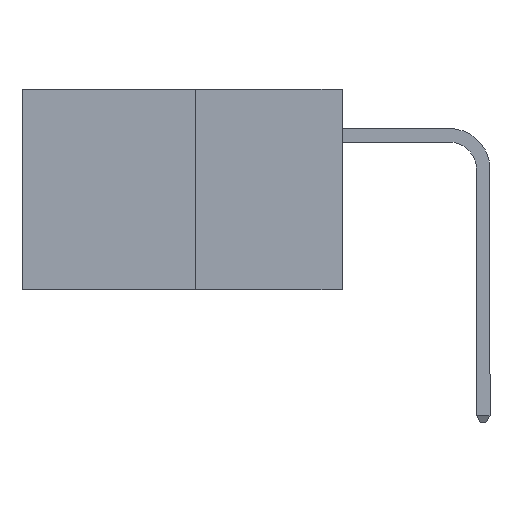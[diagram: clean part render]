
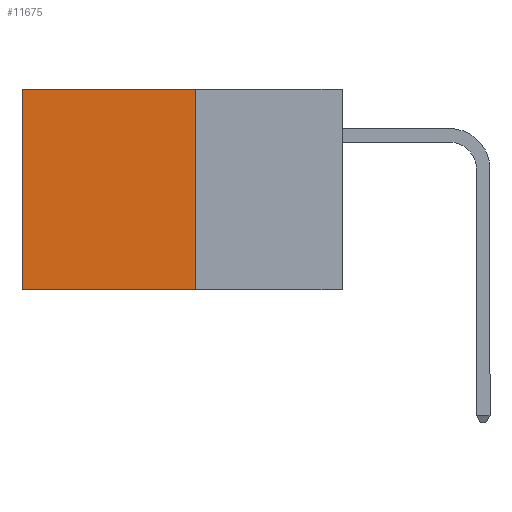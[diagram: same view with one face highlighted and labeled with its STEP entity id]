
A CAD part, left-side view. The second image highlights one B-rep face of the part: STEP entity #11675.
In plain terms, the highlighted planar face has unit normal (-1, 0, 0).
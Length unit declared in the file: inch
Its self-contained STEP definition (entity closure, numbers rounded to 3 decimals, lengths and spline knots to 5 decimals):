
#124 = LINE ( 'NONE', #11530, #7483 ) ;
#128 = CARTESIAN_POINT ( 'NONE',  ( 0.277, 0.59, -0.37 ) ) ;
#208 = VERTEX_POINT ( 'NONE', #7636 ) ;
#1012 = CARTESIAN_POINT ( 'NONE',  ( 0.277, 0.59, 0. ) ) ;
#1366 = ORIENTED_EDGE ( 'NONE', *, *, #8834, .T. ) ;
#1593 = CARTESIAN_POINT ( 'NONE',  ( 0.277, 0.27, -0.37 ) ) ;
#1611 = DIRECTION ( 'NONE',  ( 0., 1., 0. ) ) ;
#2926 = DIRECTION ( 'NONE',  ( 0., 0., -1. ) ) ;
#3081 = VERTEX_POINT ( 'NONE', #1012 ) ;
#3331 = ORIENTED_EDGE ( 'NONE', *, *, #4728, .F. ) ;
#4112 = DIRECTION ( 'NONE',  ( 0., 0., -1. ) ) ;
#4430 = FACE_OUTER_BOUND ( 'NONE', #7140, .T. ) ;
#4728 = EDGE_CURVE ( 'NONE', #208, #9255, #12239, .T. ) ;
#5183 = EDGE_CURVE ( 'NONE', #6475, #208, #7629, .T. ) ;
#5600 = ORIENTED_EDGE ( 'NONE', *, *, #7944, .T. ) ;
#5787 = CARTESIAN_POINT ( 'NONE',  ( 0.277, 0.27, 0. ) ) ;
#6002 = AXIS2_PLACEMENT_3D ( 'NONE', #6958, #9772, #4112 ) ;
#6021 = PLANE ( 'NONE',  #6002 ) ;
#6188 = ORIENTED_EDGE ( 'NONE', *, *, #5183, .F. ) ;
#6475 = VERTEX_POINT ( 'NONE', #5787 ) ;
#6736 = CARTESIAN_POINT ( 'NONE',  ( 0.277, 0.27, -0.37 ) ) ;
#6958 = CARTESIAN_POINT ( 'NONE',  ( 0.277, 0.27, -0.37 ) ) ;
#7140 = EDGE_LOOP ( 'NONE', ( #5600, #3331, #6188, #1366 ) ) ;
#7326 = VECTOR ( 'NONE', #2926, 39.37008 ) ;
#7483 = VECTOR ( 'NONE', #11489, 39.37008 ) ;
#7629 = LINE ( 'NONE', #6736, #7326 ) ;
#7636 = CARTESIAN_POINT ( 'NONE',  ( 0.277, 0.27, -0.37 ) ) ;
#7944 = EDGE_CURVE ( 'NONE', #3081, #9255, #11169, .T. ) ;
#8469 = CARTESIAN_POINT ( 'NONE',  ( 0.277, 0.59, -0.37 ) ) ;
#8718 = VECTOR ( 'NONE', #11247, 39.37008 ) ;
#8834 = EDGE_CURVE ( 'NONE', #6475, #3081, #124, .T. ) ;
#9255 = VERTEX_POINT ( 'NONE', #128 ) ;
#9772 = DIRECTION ( 'NONE',  ( 1., 0., 0. ) ) ;
#9814 = VECTOR ( 'NONE', #1611, 39.37008 ) ;
#11169 = LINE ( 'NONE', #8469, #8718 ) ;
#11247 = DIRECTION ( 'NONE',  ( 0., 0., -1. ) ) ;
#11489 = DIRECTION ( 'NONE',  ( 0., 1., 0. ) ) ;
#11530 = CARTESIAN_POINT ( 'NONE',  ( 0.277, 0.27, 0. ) ) ;
#11675 = ADVANCED_FACE ( 'NONE', ( #4430 ), #6021, .F. ) ;
#12239 = LINE ( 'NONE', #1593, #9814 ) ;
